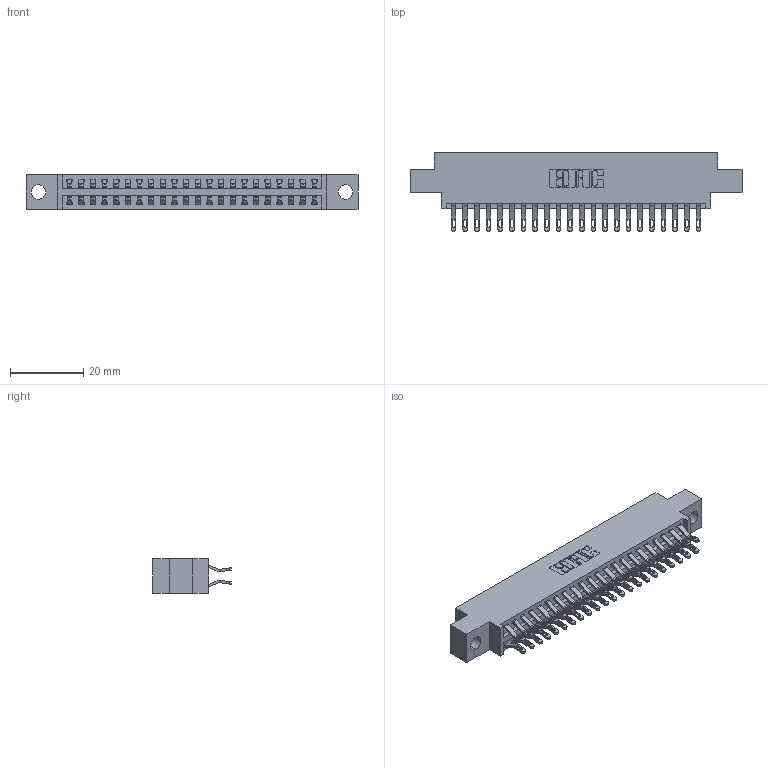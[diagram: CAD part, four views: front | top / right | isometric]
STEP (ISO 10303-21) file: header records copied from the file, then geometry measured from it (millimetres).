
FILE_DESCRIPTION (( 'STEP AP203' ), '1' );
FILE_NAME ('346-044-555-804.STEP', '2022-05-20T07:42:19', ( '' ), ( '' ), 'SwSTEP 2.0', 'SolidWorks 2020', '' );
FILE_SCHEMA (( 'CONFIG_CONTROL_DESIGN' ));
Length unit declared in the file: inch
Products named in the file (3): 346 Part_0.170 Offset - 0.156 Dia-TH; 346-044-555-804; 345-292-001_555 Tail
Assembly tree (45 placements, depth 2):
  346-044-555-804
    346 Part_0.170 Offset - 0.156 Dia-TH
    345-292-001_555 Tail  x44
Bounding box: 90.42 x 21.46 x 9.4 mm (x, y, z)
Volume: 8529.2 mm3; surface area: 11892 mm2
Topology: 45 solids, 45 shells, 2692 faces, 8429 edges, 5618 vertices
Faces by surface type: plane 1546, cylinder 1146
Entity records: 17927 total; most frequent: CARTESIAN_POINT 3024, ORIENTED_EDGE 2926, DIRECTION 2683, EDGE_CURVE 1463, LINE 1223, VECTOR 1223, VERTEX_POINT 974, AXIS2_PLACEMENT_3D 730
